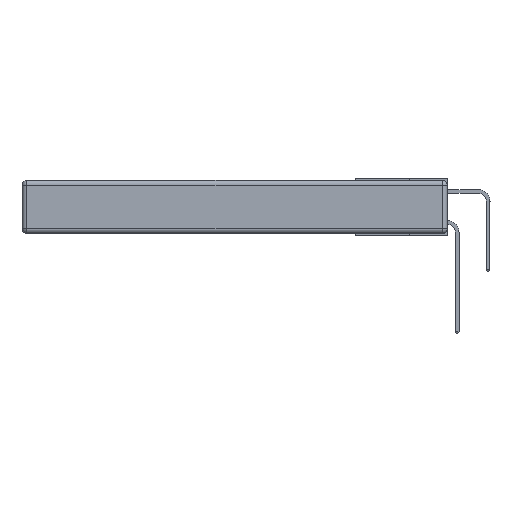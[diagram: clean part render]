
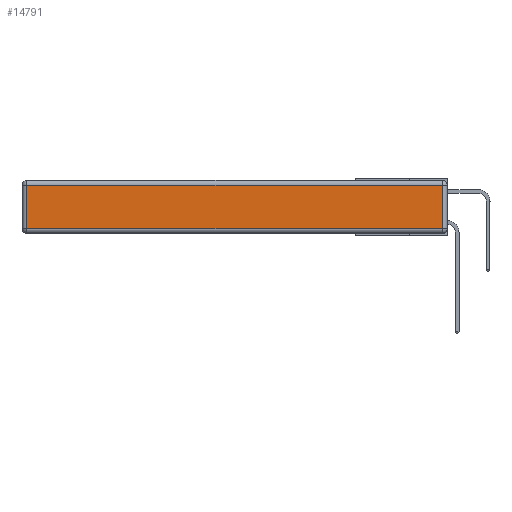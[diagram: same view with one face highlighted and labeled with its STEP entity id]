
A CAD part, left-side view. The second image highlights one B-rep face of the part: STEP entity #14791.
In plain terms, the highlighted planar face has unit normal (-1, 0, 0).
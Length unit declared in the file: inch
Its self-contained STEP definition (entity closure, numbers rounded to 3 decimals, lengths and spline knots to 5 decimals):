
#92 = CARTESIAN_POINT ( 'NONE',  ( 0., 0.03, -0.343 ) ) ;
#385 = ORIENTED_EDGE ( 'NONE', *, *, #14179, .T. ) ;
#936 = LINE ( 'NONE', #92, #11231 ) ;
#1359 = DIRECTION ( 'NONE',  ( 0., 0., 1. ) ) ;
#1458 = DIRECTION ( 'NONE',  ( 0., 0., 1. ) ) ;
#1930 = VERTEX_POINT ( 'NONE', #12957 ) ;
#3466 = DIRECTION ( 'NONE',  ( 0., 0., -1. ) ) ;
#5553 = PLANE ( 'NONE',  #7598 ) ;
#5934 = EDGE_CURVE ( 'NONE', #10499, #12984, #12063, .T. ) ;
#6832 = EDGE_LOOP ( 'NONE', ( #13167, #7040, #16969, #385 ) ) ;
#7032 = EDGE_CURVE ( 'NONE', #1930, #11464, #10300, .T. ) ;
#7040 = ORIENTED_EDGE ( 'NONE', *, *, #9604, .T. ) ;
#7598 = AXIS2_PLACEMENT_3D ( 'NONE', #9568, #8304, #1359 ) ;
#8304 = DIRECTION ( 'NONE',  ( -1., 0., 0. ) ) ;
#8420 = VECTOR ( 'NONE', #16246, 39.37008 ) ;
#9342 = VECTOR ( 'NONE', #3466, 39.37008 ) ;
#9568 = CARTESIAN_POINT ( 'NONE',  ( 0., 0., -0.343 ) ) ;
#9604 = EDGE_CURVE ( 'NONE', #11464, #10499, #936, .T. ) ;
#10300 = LINE ( 'NONE', #15778, #12649 ) ;
#10499 = VERTEX_POINT ( 'NONE', #12755 ) ;
#11231 = VECTOR ( 'NONE', #1458, 39.37008 ) ;
#11464 = VERTEX_POINT ( 'NONE', #12105 ) ;
#12063 = LINE ( 'NONE', #16377, #8420 ) ;
#12105 = CARTESIAN_POINT ( 'NONE',  ( 0., 0.03, -0.313 ) ) ;
#12649 = VECTOR ( 'NONE', #15835, 39.37008 ) ;
#12755 = CARTESIAN_POINT ( 'NONE',  ( 0., 0.03, -0.03 ) ) ;
#12827 = CARTESIAN_POINT ( 'NONE',  ( 0., 2.72, -0.343 ) ) ;
#12957 = CARTESIAN_POINT ( 'NONE',  ( 0., 2.72, -0.313 ) ) ;
#12984 = VERTEX_POINT ( 'NONE', #13423 ) ;
#13167 = ORIENTED_EDGE ( 'NONE', *, *, #7032, .T. ) ;
#13423 = CARTESIAN_POINT ( 'NONE',  ( 0., 2.72, -0.03 ) ) ;
#14038 = FACE_OUTER_BOUND ( 'NONE', #6832, .T. ) ;
#14179 = EDGE_CURVE ( 'NONE', #12984, #1930, #17479, .T. ) ;
#14791 = ADVANCED_FACE ( 'NONE', ( #14038 ), #5553, .T. ) ;
#15778 = CARTESIAN_POINT ( 'NONE',  ( 0., 0., -0.313 ) ) ;
#15835 = DIRECTION ( 'NONE',  ( 0., -1., 0. ) ) ;
#16246 = DIRECTION ( 'NONE',  ( 0., 1., 0. ) ) ;
#16377 = CARTESIAN_POINT ( 'NONE',  ( 0., 2.75, -0.03 ) ) ;
#16969 = ORIENTED_EDGE ( 'NONE', *, *, #5934, .T. ) ;
#17479 = LINE ( 'NONE', #12827, #9342 ) ;
